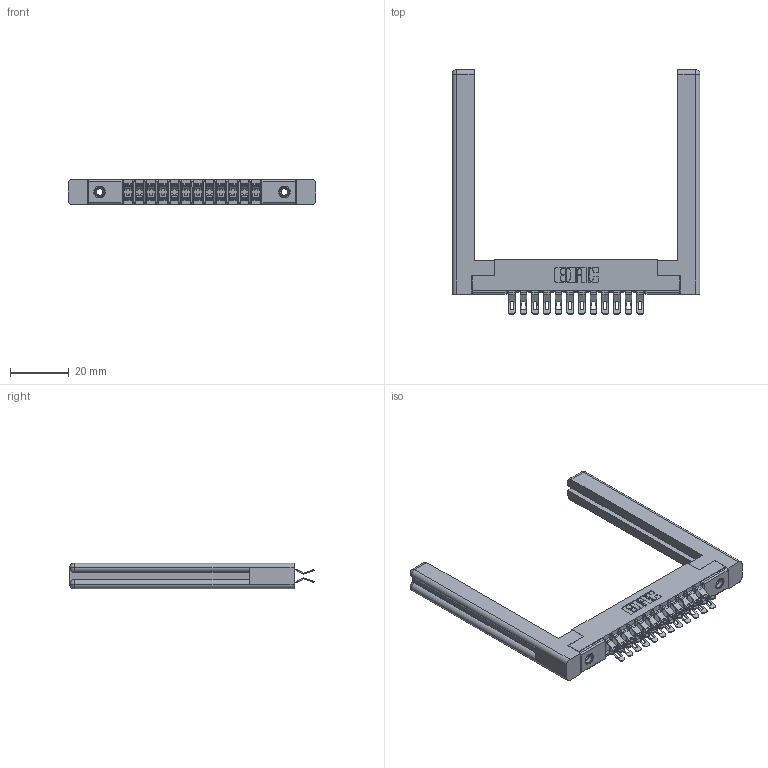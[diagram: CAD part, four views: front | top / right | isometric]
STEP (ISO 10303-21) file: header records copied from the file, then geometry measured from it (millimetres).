
FILE_DESCRIPTION (( 'STEP AP203' ), '1' );
FILE_NAME ('307-024-455-258.STEP', '2020-09-29T05:17:44', ( '' ), ( '' ), 'SwSTEP 2.0', 'SolidWorks 2020', '' );
FILE_SCHEMA (( 'CONFIG_CONTROL_DESIGN' ));
Length unit declared in the file: inch
Products named in the file (5): 307-220-058; 307-024-455-258; 307 Part_.156 Dia Mounting Holes; 307-290-001_555; 345-250-001_345-250-001-102
Assembly tree (29 placements, depth 2):
  307-024-455-258
    307 Part_.156 Dia Mounting Holes
    307-290-001_555  x24
    307-220-058  x2
    345-250-001_345-250-001-102  x2
Bounding box: 84.18 x 83.06 x 8.71 mm (x, y, z)
Volume: 13265.2 mm3; surface area: 14816.1 mm2
Topology: 29 solids, 29 shells, 1737 faces, 5021 edges, 3266 vertices
Faces by surface type: plane 970, cylinder 717, sphere 26, torus 12, cone 12
Entity records: 17540 total; most frequent: CARTESIAN_POINT 2903, DIRECTION 2821, ORIENTED_EDGE 2818, EDGE_CURVE 1409, VECTOR 1053, LINE 1053, VERTEX_POINT 912, AXIS2_PLACEMENT_3D 884
